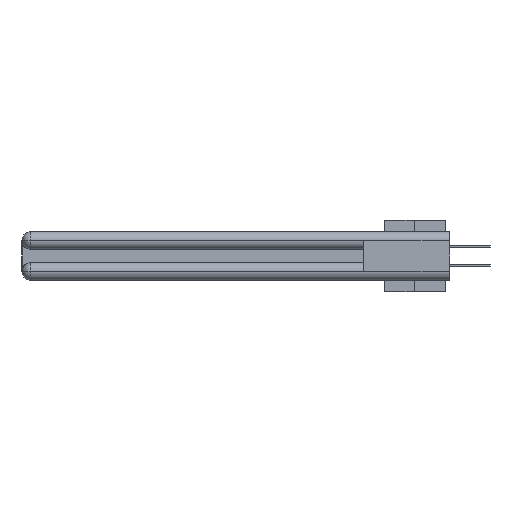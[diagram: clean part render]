
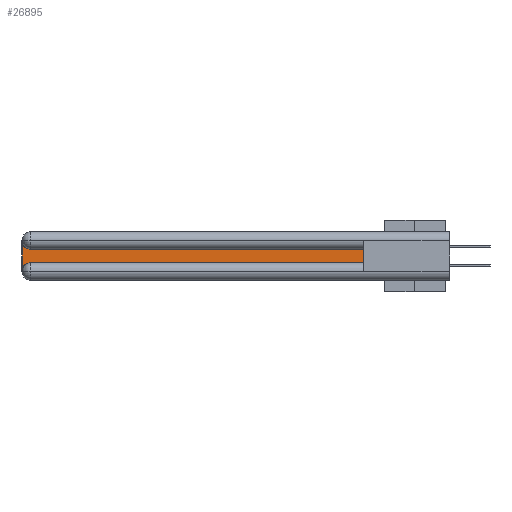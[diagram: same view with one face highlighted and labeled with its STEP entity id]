
A CAD part, left-side view. The second image highlights one B-rep face of the part: STEP entity #26895.
In plain terms, the highlighted planar face has unit normal (-1, 0, 0).
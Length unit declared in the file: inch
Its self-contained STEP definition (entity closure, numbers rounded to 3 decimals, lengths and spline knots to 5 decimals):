
#1807 = VERTEX_POINT ( 'NONE', #15954 ) ;
#2151 = CARTESIAN_POINT ( 'NONE',  ( 0.075, 2.94, -0.2175 ) ) ;
#2835 = LINE ( 'NONE', #10214, #9141 ) ;
#4080 = ORIENTED_EDGE ( 'NONE', *, *, #29538, .T. ) ;
#4088 = CIRCLE ( 'NONE', #40850, 0.06 ) ;
#4443 = VERTEX_POINT ( 'NONE', #30214 ) ;
#4462 = EDGE_CURVE ( 'NONE', #26300, #35788, #2835, .T. ) ;
#7048 = LINE ( 'NONE', #9711, #23271 ) ;
#8144 = CIRCLE ( 'NONE', #33075, 0.06 ) ;
#9141 = VECTOR ( 'NONE', #20614, 39.37008 ) ;
#9509 = EDGE_CURVE ( 'NONE', #1807, #26300, #4088, .T. ) ;
#9711 = CARTESIAN_POINT ( 'NONE',  ( 0.075, 0.6, -0.2175 ) ) ;
#10214 = CARTESIAN_POINT ( 'NONE',  ( 0.075, 3., -0.2175 ) ) ;
#11327 = DIRECTION ( 'NONE',  ( 1., 0., 0. ) ) ;
#11662 = VERTEX_POINT ( 'NONE', #2151 ) ;
#13855 = CARTESIAN_POINT ( 'NONE',  ( 0.075, 2.94, -0.2775 ) ) ;
#14653 = DIRECTION ( 'NONE',  ( 0., 0., -1. ) ) ;
#14883 = LINE ( 'NONE', #32537, #41562 ) ;
#15692 = DIRECTION ( 'NONE',  ( 0., 1., 0. ) ) ;
#15954 = CARTESIAN_POINT ( 'NONE',  ( 0.075, 2.94, -0.1225 ) ) ;
#17182 = LINE ( 'NONE', #21878, #21455 ) ;
#17799 = DIRECTION ( 'NONE',  ( 0., 0., -1. ) ) ;
#19347 = EDGE_LOOP ( 'NONE', ( #38078, #41122, #39509, #4080, #40937, #35466 ) ) ;
#20475 = DIRECTION ( 'NONE',  ( 0., 0., -1. ) ) ;
#20614 = DIRECTION ( 'NONE',  ( 0., 0., -1. ) ) ;
#21455 = VECTOR ( 'NONE', #28025, 39.37008 ) ;
#21878 = CARTESIAN_POINT ( 'NONE',  ( 0.075, 0.6, -0.2175 ) ) ;
#23271 = VECTOR ( 'NONE', #27558, 39.37008 ) ;
#23355 = FACE_OUTER_BOUND ( 'NONE', #19347, .T. ) ;
#24128 = DIRECTION ( 'NONE',  ( 1., 0., 0. ) ) ;
#25685 = EDGE_CURVE ( 'NONE', #11662, #29225, #17182, .T. ) ;
#26300 = VERTEX_POINT ( 'NONE', #31083 ) ;
#26895 = ADVANCED_FACE ( 'NONE', ( #23355 ), #33884, .F. ) ;
#27558 = DIRECTION ( 'NONE',  ( 0., 0., 1. ) ) ;
#28025 = DIRECTION ( 'NONE',  ( 0., -1., 0. ) ) ;
#29225 = VERTEX_POINT ( 'NONE', #39758 ) ;
#29366 = AXIS2_PLACEMENT_3D ( 'NONE', #37253, #40627, #17799 ) ;
#29538 = EDGE_CURVE ( 'NONE', #35788, #11662, #8144, .T. ) ;
#29956 = EDGE_CURVE ( 'NONE', #29225, #4443, #7048, .T. ) ;
#30214 = CARTESIAN_POINT ( 'NONE',  ( 0.075, 0.6, -0.1225 ) ) ;
#31083 = CARTESIAN_POINT ( 'NONE',  ( 0.075, 3., -0.0625 ) ) ;
#32537 = CARTESIAN_POINT ( 'NONE',  ( 0.075, 0.6, -0.1225 ) ) ;
#33075 = AXIS2_PLACEMENT_3D ( 'NONE', #13855, #24128, #20475 ) ;
#33884 = PLANE ( 'NONE',  #29366 ) ;
#35466 = ORIENTED_EDGE ( 'NONE', *, *, #29956, .T. ) ;
#35788 = VERTEX_POINT ( 'NONE', #39143 ) ;
#37253 = CARTESIAN_POINT ( 'NONE',  ( 0.075, 3., -0.1225 ) ) ;
#37924 = CARTESIAN_POINT ( 'NONE',  ( 0.075, 2.94, -0.0625 ) ) ;
#38078 = ORIENTED_EDGE ( 'NONE', *, *, #41590, .T. ) ;
#39143 = CARTESIAN_POINT ( 'NONE',  ( 0.075, 3., -0.2775 ) ) ;
#39509 = ORIENTED_EDGE ( 'NONE', *, *, #4462, .T. ) ;
#39758 = CARTESIAN_POINT ( 'NONE',  ( 0.075, 0.6, -0.2175 ) ) ;
#40627 = DIRECTION ( 'NONE',  ( 1., 0., 0. ) ) ;
#40850 = AXIS2_PLACEMENT_3D ( 'NONE', #37924, #11327, #14653 ) ;
#40937 = ORIENTED_EDGE ( 'NONE', *, *, #25685, .T. ) ;
#41122 = ORIENTED_EDGE ( 'NONE', *, *, #9509, .T. ) ;
#41562 = VECTOR ( 'NONE', #15692, 39.37008 ) ;
#41590 = EDGE_CURVE ( 'NONE', #4443, #1807, #14883, .T. ) ;
